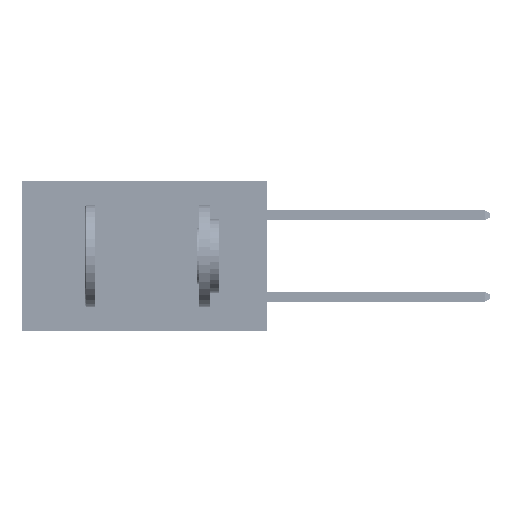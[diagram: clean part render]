
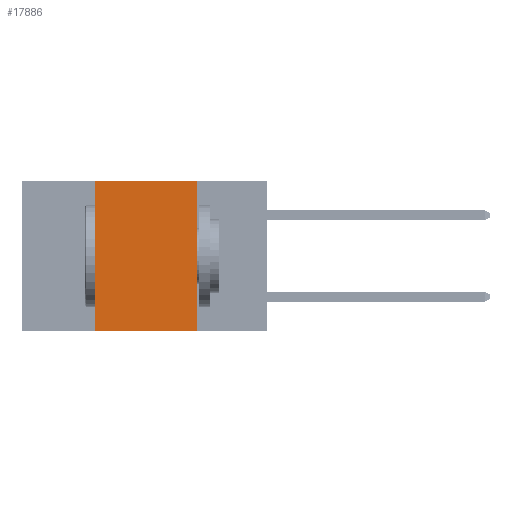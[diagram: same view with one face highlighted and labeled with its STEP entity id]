
A CAD part, left-side view. The second image highlights one B-rep face of the part: STEP entity #17886.
In plain terms, the highlighted planar face has unit normal (-1, 0, 0).
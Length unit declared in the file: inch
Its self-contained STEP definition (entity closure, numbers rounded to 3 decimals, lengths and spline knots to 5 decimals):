
#2142 = DIRECTION ( 'NONE',  ( 0., 0., -1. ) ) ;
#6178 = ORIENTED_EDGE ( 'NONE', *, *, #17618, .F. ) ;
#9359 = CARTESIAN_POINT ( 'NONE',  ( 0., 0.42, 0. ) ) ;
#9600 = EDGE_LOOP ( 'NONE', ( #14920, #6178, #20723, #11605 ) ) ;
#11495 = DIRECTION ( 'NONE',  ( 0., -1., 0. ) ) ;
#11605 = ORIENTED_EDGE ( 'NONE', *, *, #38794, .T. ) ;
#12962 = VERTEX_POINT ( 'NONE', #23315 ) ;
#14920 = ORIENTED_EDGE ( 'NONE', *, *, #18659, .F. ) ;
#16363 = VECTOR ( 'NONE', #24128, 39.37008 ) ;
#17618 = EDGE_CURVE ( 'NONE', #35038, #44619, #33587, .T. ) ;
#17886 = ADVANCED_FACE ( 'NONE', ( #18091 ), #39992, .F. ) ;
#18091 = FACE_OUTER_BOUND ( 'NONE', #9600, .T. ) ;
#18659 = EDGE_CURVE ( 'NONE', #44619, #29326, #24002, .T. ) ;
#18753 = CARTESIAN_POINT ( 'NONE',  ( 0., 0.6, -0.37 ) ) ;
#20723 = ORIENTED_EDGE ( 'NONE', *, *, #22614, .F. ) ;
#20927 = DIRECTION ( 'NONE',  ( 0., 0., -1. ) ) ;
#22614 = EDGE_CURVE ( 'NONE', #12962, #35038, #41708, .T. ) ;
#22649 = LINE ( 'NONE', #18753, #23879 ) ;
#23315 = CARTESIAN_POINT ( 'NONE',  ( 0., 0.42, -0.37 ) ) ;
#23879 = VECTOR ( 'NONE', #11495, 39.37008 ) ;
#24002 = LINE ( 'NONE', #33329, #34206 ) ;
#24128 = DIRECTION ( 'NONE',  ( 0., 0., 1. ) ) ;
#24610 = VECTOR ( 'NONE', #45923, 39.37008 ) ;
#26255 = CARTESIAN_POINT ( 'NONE',  ( 0., 0.17, -0.37 ) ) ;
#28701 = DIRECTION ( 'NONE',  ( 1., 0., 0. ) ) ;
#29326 = VERTEX_POINT ( 'NONE', #26255 ) ;
#31346 = CARTESIAN_POINT ( 'NONE',  ( 0., 0.42, 0. ) ) ;
#33329 = CARTESIAN_POINT ( 'NONE',  ( 0., 0.17, 0. ) ) ;
#33587 = LINE ( 'NONE', #34745, #24610 ) ;
#34206 = VECTOR ( 'NONE', #2142, 39.37008 ) ;
#34745 = CARTESIAN_POINT ( 'NONE',  ( 0., 0.6, 0. ) ) ;
#35038 = VERTEX_POINT ( 'NONE', #9359 ) ;
#36857 = AXIS2_PLACEMENT_3D ( 'NONE', #47606, #28701, #20927 ) ;
#38289 = CARTESIAN_POINT ( 'NONE',  ( 0., 0.17, 0. ) ) ;
#38794 = EDGE_CURVE ( 'NONE', #12962, #29326, #22649, .T. ) ;
#39992 = PLANE ( 'NONE',  #36857 ) ;
#41708 = LINE ( 'NONE', #31346, #16363 ) ;
#44619 = VERTEX_POINT ( 'NONE', #38289 ) ;
#45923 = DIRECTION ( 'NONE',  ( 0., -1., 0. ) ) ;
#47606 = CARTESIAN_POINT ( 'NONE',  ( 0., 0.6, 0. ) ) ;
